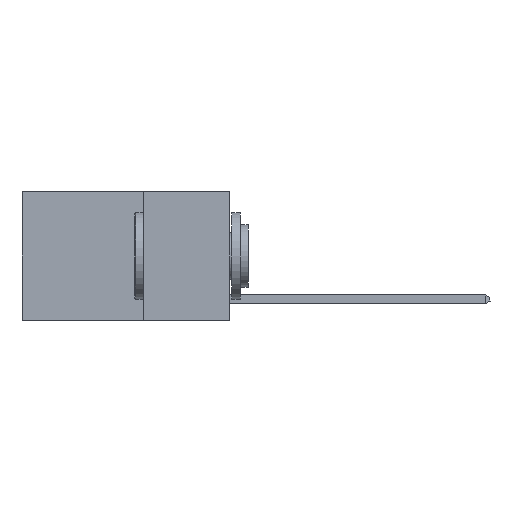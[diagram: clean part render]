
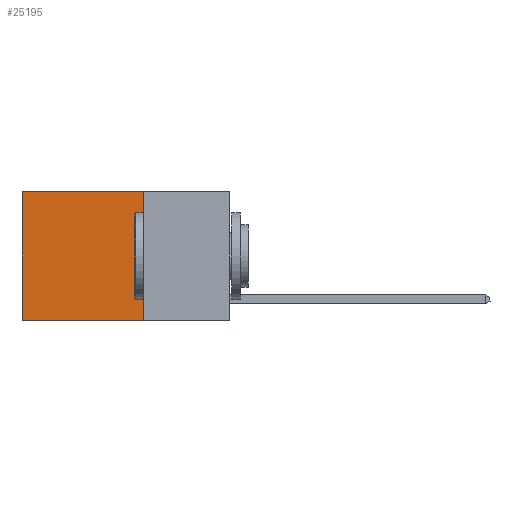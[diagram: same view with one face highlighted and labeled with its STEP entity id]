
A CAD part, left-side view. The second image highlights one B-rep face of the part: STEP entity #25195.
In plain terms, the highlighted planar face has unit normal (-1, 0, 0).
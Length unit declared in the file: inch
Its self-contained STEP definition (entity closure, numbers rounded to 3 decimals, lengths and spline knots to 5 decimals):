
#41 = CARTESIAN_POINT ( 'NONE',  ( 0.2625, 0.25, 0. ) ) ;
#532 = VERTEX_POINT ( 'NONE', #3657 ) ;
#1283 = CARTESIAN_POINT ( 'NONE',  ( 0.2625, 0.25, 0. ) ) ;
#1568 = EDGE_CURVE ( 'NONE', #26081, #28433, #4281, .T. ) ;
#1629 = LINE ( 'NONE', #23251, #12769 ) ;
#2055 = LINE ( 'NONE', #21603, #24996 ) ;
#2261 = DIRECTION ( 'NONE',  ( 0., 0., -1. ) ) ;
#3127 = EDGE_CURVE ( 'NONE', #532, #26081, #2055, .T. ) ;
#3657 = CARTESIAN_POINT ( 'NONE',  ( 0.2625, 0.25, 0. ) ) ;
#4281 = LINE ( 'NONE', #9614, #14699 ) ;
#4736 = AXIS2_PLACEMENT_3D ( 'NONE', #41, #15607, #2261 ) ;
#5727 = CARTESIAN_POINT ( 'NONE',  ( 0.2625, 0.6, 0. ) ) ;
#9614 = CARTESIAN_POINT ( 'NONE',  ( 0.2625, 0.6, 0. ) ) ;
#11852 = DIRECTION ( 'NONE',  ( 0., 0., -1. ) ) ;
#12748 = DIRECTION ( 'NONE',  ( 0., 1., 0. ) ) ;
#12769 = VECTOR ( 'NONE', #25451, 39.37008 ) ;
#13358 = PLANE ( 'NONE',  #4736 ) ;
#14699 = VECTOR ( 'NONE', #11852, 39.37008 ) ;
#15471 = ORIENTED_EDGE ( 'NONE', *, *, #19385, .F. ) ;
#15607 = DIRECTION ( 'NONE',  ( 1., 0., 0. ) ) ;
#16917 = FACE_OUTER_BOUND ( 'NONE', #27156, .T. ) ;
#18685 = ORIENTED_EDGE ( 'NONE', *, *, #26775, .F. ) ;
#18765 = CARTESIAN_POINT ( 'NONE',  ( 0.2625, 0.6, -0.37 ) ) ;
#18886 = ORIENTED_EDGE ( 'NONE', *, *, #3127, .T. ) ;
#19385 = EDGE_CURVE ( 'NONE', #27120, #28433, #1629, .T. ) ;
#19616 = VECTOR ( 'NONE', #25662, 39.37008 ) ;
#20213 = CARTESIAN_POINT ( 'NONE',  ( 0.2625, 0.25, -0.37 ) ) ;
#20990 = LINE ( 'NONE', #1283, #19616 ) ;
#21603 = CARTESIAN_POINT ( 'NONE',  ( 0.2625, 0.25, 0. ) ) ;
#23251 = CARTESIAN_POINT ( 'NONE',  ( 0.2625, 0.25, -0.37 ) ) ;
#23479 = ORIENTED_EDGE ( 'NONE', *, *, #1568, .T. ) ;
#24996 = VECTOR ( 'NONE', #12748, 39.37008 ) ;
#25195 = ADVANCED_FACE ( 'NONE', ( #16917 ), #13358, .F. ) ;
#25451 = DIRECTION ( 'NONE',  ( 0., 1., 0. ) ) ;
#25662 = DIRECTION ( 'NONE',  ( 0., 0., -1. ) ) ;
#26081 = VERTEX_POINT ( 'NONE', #5727 ) ;
#26775 = EDGE_CURVE ( 'NONE', #532, #27120, #20990, .T. ) ;
#27120 = VERTEX_POINT ( 'NONE', #20213 ) ;
#27156 = EDGE_LOOP ( 'NONE', ( #23479, #15471, #18685, #18886 ) ) ;
#28433 = VERTEX_POINT ( 'NONE', #18765 ) ;
